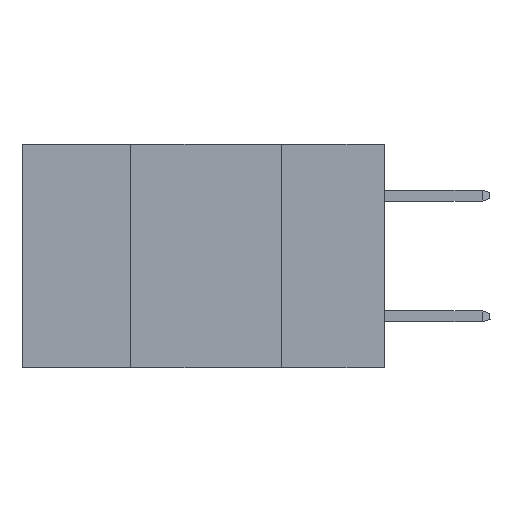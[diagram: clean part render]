
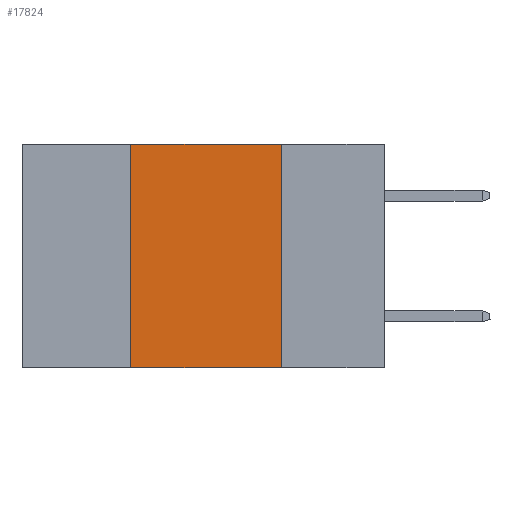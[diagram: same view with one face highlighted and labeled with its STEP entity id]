
A CAD part, left-side view. The second image highlights one B-rep face of the part: STEP entity #17824.
In plain terms, the highlighted planar face has unit normal (-1, 0, 0).
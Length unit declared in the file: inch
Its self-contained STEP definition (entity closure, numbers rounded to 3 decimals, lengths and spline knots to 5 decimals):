
#1506 = CARTESIAN_POINT ( 'NONE',  ( 0., 0.6, -0.37 ) ) ;
#1790 = DIRECTION ( 'NONE',  ( 0., 0., -1. ) ) ;
#1877 = CARTESIAN_POINT ( 'NONE',  ( 0., 0.17, -0.37 ) ) ;
#2232 = CARTESIAN_POINT ( 'NONE',  ( 0., 0.17, 0. ) ) ;
#2813 = EDGE_CURVE ( 'NONE', #6413, #20109, #9057, .T. ) ;
#2818 = FACE_OUTER_BOUND ( 'NONE', #22885, .T. ) ;
#4437 = AXIS2_PLACEMENT_3D ( 'NONE', #8048, #8142, #21739 ) ;
#5099 = LINE ( 'NONE', #1506, #20708 ) ;
#5870 = ORIENTED_EDGE ( 'NONE', *, *, #22907, .F. ) ;
#6197 = DIRECTION ( 'NONE',  ( 0., -1., 0. ) ) ;
#6413 = VERTEX_POINT ( 'NONE', #2232 ) ;
#7087 = VECTOR ( 'NONE', #6197, 39.37008 ) ;
#8048 = CARTESIAN_POINT ( 'NONE',  ( 0., 0.6, 0. ) ) ;
#8142 = DIRECTION ( 'NONE',  ( 1., 0., 0. ) ) ;
#8348 = LINE ( 'NONE', #16043, #7087 ) ;
#9057 = LINE ( 'NONE', #1877, #18818 ) ;
#9834 = VERTEX_POINT ( 'NONE', #13567 ) ;
#11120 = VERTEX_POINT ( 'NONE', #21423 ) ;
#11217 = ORIENTED_EDGE ( 'NONE', *, *, #12576, .T. ) ;
#12576 = EDGE_CURVE ( 'NONE', #11120, #20109, #5099, .T. ) ;
#12786 = LINE ( 'NONE', #15943, #21863 ) ;
#13567 = CARTESIAN_POINT ( 'NONE',  ( 0., 0.42, 0. ) ) ;
#15353 = DIRECTION ( 'NONE',  ( 0., -1., 0. ) ) ;
#15943 = CARTESIAN_POINT ( 'NONE',  ( 0., 0.42, -0.37 ) ) ;
#16043 = CARTESIAN_POINT ( 'NONE',  ( 0., 0.6, 0. ) ) ;
#16544 = EDGE_CURVE ( 'NONE', #11120, #9834, #12786, .T. ) ;
#17824 = ADVANCED_FACE ( 'NONE', ( #2818 ), #19830, .F. ) ;
#17871 = DIRECTION ( 'NONE',  ( 0., 0., 1. ) ) ;
#17979 = CARTESIAN_POINT ( 'NONE',  ( 0., 0.17, -0.37 ) ) ;
#18818 = VECTOR ( 'NONE', #1790, 39.37008 ) ;
#19830 = PLANE ( 'NONE',  #4437 ) ;
#20109 = VERTEX_POINT ( 'NONE', #17979 ) ;
#20708 = VECTOR ( 'NONE', #15353, 39.37008 ) ;
#21423 = CARTESIAN_POINT ( 'NONE',  ( 0., 0.42, -0.37 ) ) ;
#21739 = DIRECTION ( 'NONE',  ( 0., 0., -1. ) ) ;
#21863 = VECTOR ( 'NONE', #17871, 39.37008 ) ;
#22366 = ORIENTED_EDGE ( 'NONE', *, *, #16544, .F. ) ;
#22885 = EDGE_LOOP ( 'NONE', ( #23750, #5870, #22366, #11217 ) ) ;
#22907 = EDGE_CURVE ( 'NONE', #9834, #6413, #8348, .T. ) ;
#23750 = ORIENTED_EDGE ( 'NONE', *, *, #2813, .F. ) ;
